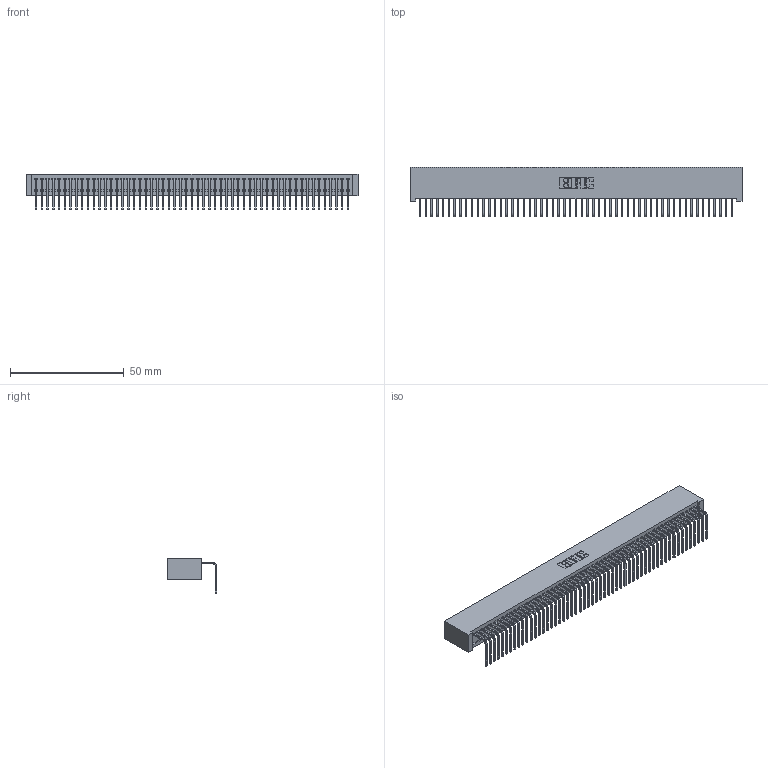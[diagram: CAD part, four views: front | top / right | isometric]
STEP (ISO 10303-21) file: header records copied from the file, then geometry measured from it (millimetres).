
FILE_DESCRIPTION (( 'STEP AP203' ), '1' );
FILE_NAME ('342-055-558-101.STEP', '2019-10-03T04:19:15', ( '' ), ( '' ), 'SwSTEP 2.0', 'SolidWorks 2016', '' );
FILE_SCHEMA (( 'CONFIG_CONTROL_DESIGN' ));
Length unit declared in the file: inch
Products named in the file (3): 345-292-001_558 Tail - 2; 342-055-558-101; 342 Part_Lugless
Assembly tree (56 placements, depth 2):
  342-055-558-101
    342 Part_Lugless
    345-292-001_558 Tail - 2  x55
Bounding box: 145.95 x 21.91 x 15.62 mm (x, y, z)
Volume: 13436.9 mm3; surface area: 21338.2 mm2
Topology: 56 solids, 56 shells, 3402 faces, 10285 edges, 6782 vertices
Faces by surface type: plane 2482, cylinder 920
Entity records: 31617 total; most frequent: CARTESIAN_POINT 5459, ORIENTED_EDGE 5450, DIRECTION 4571, EDGE_CURVE 2725, LINE 2605, VECTOR 2605, VERTEX_POINT 1814, AXIS2_PLACEMENT_3D 983
